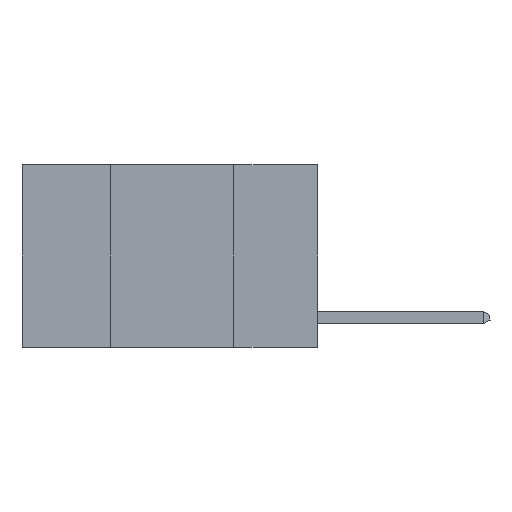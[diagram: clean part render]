
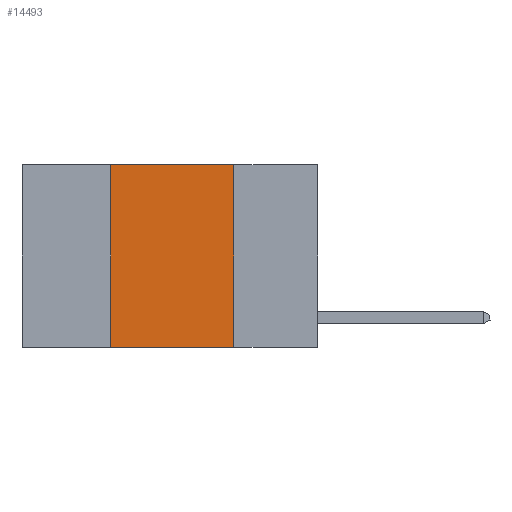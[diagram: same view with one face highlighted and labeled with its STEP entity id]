
A CAD part, left-side view. The second image highlights one B-rep face of the part: STEP entity #14493.
In plain terms, the highlighted planar face has unit normal (-1, 0, 0).
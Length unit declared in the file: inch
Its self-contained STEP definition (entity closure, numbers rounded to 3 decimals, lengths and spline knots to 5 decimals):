
#396 = EDGE_CURVE ( 'NONE', #18753, #5428, #5039, .T. ) ;
#748 = EDGE_LOOP ( 'NONE', ( #5657, #6130, #3146, #16457 ) ) ;
#981 = DIRECTION ( 'NONE',  ( 1., 0., 0. ) ) ;
#1096 = VECTOR ( 'NONE', #7793, 39.37008 ) ;
#2925 = DIRECTION ( 'NONE',  ( 0., -1., 0. ) ) ;
#3146 = ORIENTED_EDGE ( 'NONE', *, *, #9862, .F. ) ;
#3349 = CARTESIAN_POINT ( 'NONE',  ( 0., 0.42, 0. ) ) ;
#3768 = VERTEX_POINT ( 'NONE', #16238 ) ;
#3817 = CARTESIAN_POINT ( 'NONE',  ( 0., 0.6, 0. ) ) ;
#4275 = EDGE_CURVE ( 'NONE', #3768, #18753, #4443, .T. ) ;
#4329 = FACE_OUTER_BOUND ( 'NONE', #748, .T. ) ;
#4443 = LINE ( 'NONE', #16028, #15755 ) ;
#5039 = LINE ( 'NONE', #16587, #1096 ) ;
#5428 = VERTEX_POINT ( 'NONE', #9936 ) ;
#5657 = ORIENTED_EDGE ( 'NONE', *, *, #396, .F. ) ;
#5887 = LINE ( 'NONE', #3349, #10760 ) ;
#6130 = ORIENTED_EDGE ( 'NONE', *, *, #4275, .F. ) ;
#6222 = VECTOR ( 'NONE', #16015, 39.37008 ) ;
#7793 = DIRECTION ( 'NONE',  ( 0., 0., -1. ) ) ;
#8106 = CARTESIAN_POINT ( 'NONE',  ( 0., 0.17, 0. ) ) ;
#9862 = EDGE_CURVE ( 'NONE', #15314, #3768, #5887, .T. ) ;
#9936 = CARTESIAN_POINT ( 'NONE',  ( 0., 0.17, -0.37 ) ) ;
#10100 = CARTESIAN_POINT ( 'NONE',  ( 0., 0.6, -0.37 ) ) ;
#10760 = VECTOR ( 'NONE', #13700, 39.37008 ) ;
#10983 = AXIS2_PLACEMENT_3D ( 'NONE', #3817, #981, #11357 ) ;
#11357 = DIRECTION ( 'NONE',  ( 0., 0., -1. ) ) ;
#13348 = EDGE_CURVE ( 'NONE', #15314, #5428, #14052, .T. ) ;
#13700 = DIRECTION ( 'NONE',  ( 0., 0., 1. ) ) ;
#14052 = LINE ( 'NONE', #10100, #6222 ) ;
#14493 = ADVANCED_FACE ( 'NONE', ( #4329 ), #17181, .F. ) ;
#15314 = VERTEX_POINT ( 'NONE', #15881 ) ;
#15755 = VECTOR ( 'NONE', #2925, 39.37008 ) ;
#15881 = CARTESIAN_POINT ( 'NONE',  ( 0., 0.42, -0.37 ) ) ;
#16015 = DIRECTION ( 'NONE',  ( 0., -1., 0. ) ) ;
#16028 = CARTESIAN_POINT ( 'NONE',  ( 0., 0.6, 0. ) ) ;
#16238 = CARTESIAN_POINT ( 'NONE',  ( 0., 0.42, 0. ) ) ;
#16457 = ORIENTED_EDGE ( 'NONE', *, *, #13348, .T. ) ;
#16587 = CARTESIAN_POINT ( 'NONE',  ( 0., 0.17, 0. ) ) ;
#17181 = PLANE ( 'NONE',  #10983 ) ;
#18753 = VERTEX_POINT ( 'NONE', #8106 ) ;
